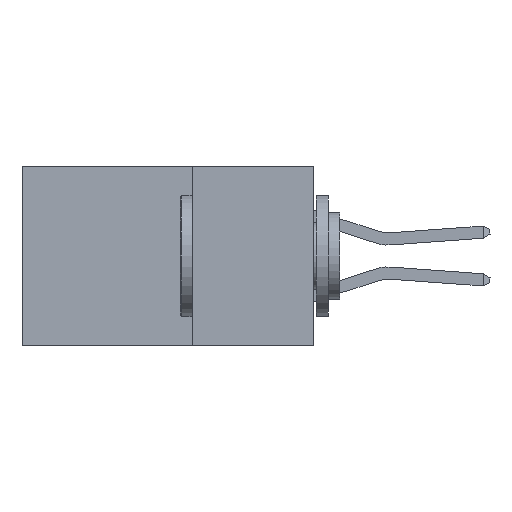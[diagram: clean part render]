
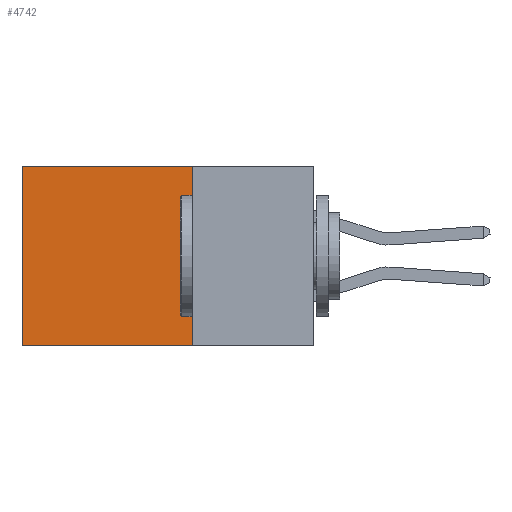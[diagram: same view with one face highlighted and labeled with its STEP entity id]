
A CAD part, left-side view. The second image highlights one B-rep face of the part: STEP entity #4742.
In plain terms, the highlighted planar face has unit normal (-1, 0, 0).
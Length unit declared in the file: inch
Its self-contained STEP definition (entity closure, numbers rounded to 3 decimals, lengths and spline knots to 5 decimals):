
#692 = CARTESIAN_POINT ( 'NONE',  ( 0.2875, 0.25, 0. ) ) ;
#785 = VECTOR ( 'NONE', #5018, 39.37008 ) ;
#951 = ORIENTED_EDGE ( 'NONE', *, *, #9407, .T. ) ;
#1333 = LINE ( 'NONE', #15252, #785 ) ;
#1385 = VECTOR ( 'NONE', #20102, 39.37008 ) ;
#1940 = DIRECTION ( 'NONE',  ( 0., 0., -1. ) ) ;
#2072 = DIRECTION ( 'NONE',  ( 1., 0., 0. ) ) ;
#2102 = DIRECTION ( 'NONE',  ( 0., 0., -1. ) ) ;
#2221 = CARTESIAN_POINT ( 'NONE',  ( 0.2875, 0.25, 0. ) ) ;
#2292 = PLANE ( 'NONE',  #19803 ) ;
#2762 = VERTEX_POINT ( 'NONE', #6232 ) ;
#3137 = EDGE_CURVE ( 'NONE', #15748, #18174, #18748, .T. ) ;
#4035 = ORIENTED_EDGE ( 'NONE', *, *, #21794, .T. ) ;
#4318 = CARTESIAN_POINT ( 'NONE',  ( 0.2875, 0.25, 0. ) ) ;
#4582 = CARTESIAN_POINT ( 'NONE',  ( 0.2875, 0.6, 0. ) ) ;
#4742 = ADVANCED_FACE ( 'NONE', ( #21541 ), #2292, .F. ) ;
#5018 = DIRECTION ( 'NONE',  ( 0., 1., 0. ) ) ;
#5785 = VERTEX_POINT ( 'NONE', #9884 ) ;
#6232 = CARTESIAN_POINT ( 'NONE',  ( 0.2875, 0.6, -0.37 ) ) ;
#6341 = DIRECTION ( 'NONE',  ( 0., 0., -1. ) ) ;
#6406 = VECTOR ( 'NONE', #6341, 39.37008 ) ;
#7300 = ORIENTED_EDGE ( 'NONE', *, *, #15348, .F. ) ;
#7403 = CARTESIAN_POINT ( 'NONE',  ( 0.2875, 0.25, -0.37 ) ) ;
#9236 = VECTOR ( 'NONE', #2102, 39.37008 ) ;
#9374 = ORIENTED_EDGE ( 'NONE', *, *, #3137, .F. ) ;
#9407 = EDGE_CURVE ( 'NONE', #5785, #2762, #19886, .T. ) ;
#9884 = CARTESIAN_POINT ( 'NONE',  ( 0.2875, 0.6, 0. ) ) ;
#15252 = CARTESIAN_POINT ( 'NONE',  ( 0.2875, 0.25, -0.37 ) ) ;
#15348 = EDGE_CURVE ( 'NONE', #18174, #2762, #1333, .T. ) ;
#15594 = LINE ( 'NONE', #18443, #1385 ) ;
#15748 = VERTEX_POINT ( 'NONE', #4318 ) ;
#17410 = EDGE_LOOP ( 'NONE', ( #951, #7300, #9374, #4035 ) ) ;
#18174 = VERTEX_POINT ( 'NONE', #7403 ) ;
#18443 = CARTESIAN_POINT ( 'NONE',  ( 0.2875, 0.25, 0. ) ) ;
#18748 = LINE ( 'NONE', #692, #9236 ) ;
#19803 = AXIS2_PLACEMENT_3D ( 'NONE', #2221, #2072, #1940 ) ;
#19886 = LINE ( 'NONE', #4582, #6406 ) ;
#20102 = DIRECTION ( 'NONE',  ( 0., 1., 0. ) ) ;
#21541 = FACE_OUTER_BOUND ( 'NONE', #17410, .T. ) ;
#21794 = EDGE_CURVE ( 'NONE', #15748, #5785, #15594, .T. ) ;
